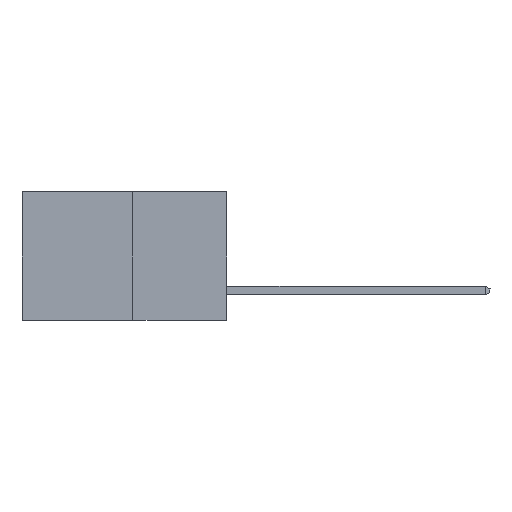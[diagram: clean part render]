
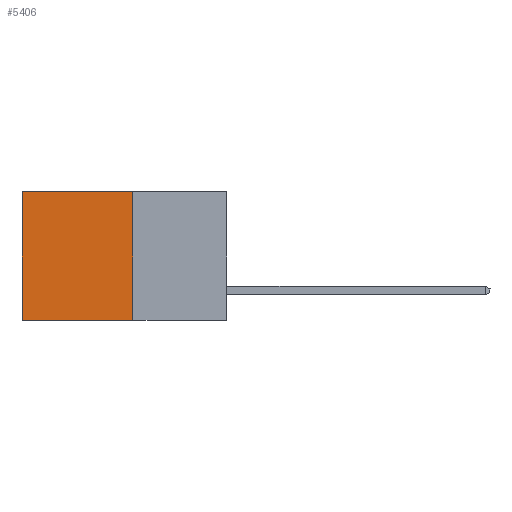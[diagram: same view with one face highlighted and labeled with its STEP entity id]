
A CAD part, left-side view. The second image highlights one B-rep face of the part: STEP entity #5406.
In plain terms, the highlighted planar face has unit normal (-1, 0, 0).
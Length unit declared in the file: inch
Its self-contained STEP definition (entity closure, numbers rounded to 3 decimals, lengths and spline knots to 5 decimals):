
#71 = VECTOR ( 'NONE', #9917, 39.37008 ) ;
#187 = CARTESIAN_POINT ( 'NONE',  ( 0.277, 0.59, 0. ) ) ;
#245 = DIRECTION ( 'NONE',  ( 0., 1., 0. ) ) ;
#254 = CARTESIAN_POINT ( 'NONE',  ( 0.277, 0.59, -0.37 ) ) ;
#568 = ORIENTED_EDGE ( 'NONE', *, *, #10129, .F. ) ;
#897 = ORIENTED_EDGE ( 'NONE', *, *, #3901, .T. ) ;
#1897 = DIRECTION ( 'NONE',  ( 0., 1., 0. ) ) ;
#2186 = LINE ( 'NONE', #2398, #11009 ) ;
#2288 = CARTESIAN_POINT ( 'NONE',  ( 0.277, 0.27, -0.37 ) ) ;
#2369 = CARTESIAN_POINT ( 'NONE',  ( 0.277, 0.27, 0. ) ) ;
#2398 = CARTESIAN_POINT ( 'NONE',  ( 0.277, 0.27, -0.37 ) ) ;
#2789 = CARTESIAN_POINT ( 'NONE',  ( 0.277, 0.27, 0. ) ) ;
#2957 = LINE ( 'NONE', #2288, #11400 ) ;
#3232 = ORIENTED_EDGE ( 'NONE', *, *, #6420, .T. ) ;
#3901 = EDGE_CURVE ( 'NONE', #10916, #3924, #14288, .T. ) ;
#3924 = VERTEX_POINT ( 'NONE', #187 ) ;
#5362 = FACE_OUTER_BOUND ( 'NONE', #14480, .T. ) ;
#5406 = ADVANCED_FACE ( 'NONE', ( #5362 ), #14065, .F. ) ;
#5822 = EDGE_CURVE ( 'NONE', #9560, #7481, #2957, .T. ) ;
#6420 = EDGE_CURVE ( 'NONE', #3924, #7481, #9271, .T. ) ;
#7481 = VERTEX_POINT ( 'NONE', #254 ) ;
#8328 = VECTOR ( 'NONE', #245, 39.37008 ) ;
#8383 = CARTESIAN_POINT ( 'NONE',  ( 0.277, 0.27, -0.37 ) ) ;
#9271 = LINE ( 'NONE', #10055, #71 ) ;
#9323 = DIRECTION ( 'NONE',  ( 0., 0., -1. ) ) ;
#9392 = ORIENTED_EDGE ( 'NONE', *, *, #5822, .F. ) ;
#9560 = VERTEX_POINT ( 'NONE', #8383 ) ;
#9917 = DIRECTION ( 'NONE',  ( 0., 0., -1. ) ) ;
#10055 = CARTESIAN_POINT ( 'NONE',  ( 0.277, 0.59, -0.37 ) ) ;
#10129 = EDGE_CURVE ( 'NONE', #10916, #9560, #2186, .T. ) ;
#10916 = VERTEX_POINT ( 'NONE', #2789 ) ;
#11009 = VECTOR ( 'NONE', #9323, 39.37008 ) ;
#11400 = VECTOR ( 'NONE', #1897, 39.37008 ) ;
#12553 = AXIS2_PLACEMENT_3D ( 'NONE', #13041, #13802, #13562 ) ;
#13041 = CARTESIAN_POINT ( 'NONE',  ( 0.277, 0.27, -0.37 ) ) ;
#13562 = DIRECTION ( 'NONE',  ( 0., 0., -1. ) ) ;
#13802 = DIRECTION ( 'NONE',  ( 1., 0., 0. ) ) ;
#14065 = PLANE ( 'NONE',  #12553 ) ;
#14288 = LINE ( 'NONE', #2369, #8328 ) ;
#14480 = EDGE_LOOP ( 'NONE', ( #3232, #9392, #568, #897 ) ) ;
